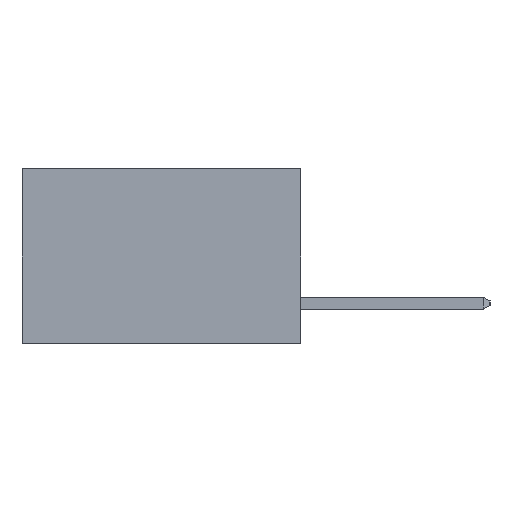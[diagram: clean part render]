
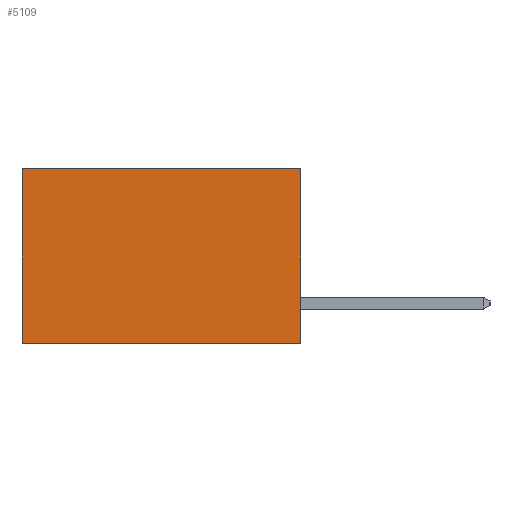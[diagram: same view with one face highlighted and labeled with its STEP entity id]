
A CAD part, left-side view. The second image highlights one B-rep face of the part: STEP entity #5109.
In plain terms, the highlighted planar face has unit normal (-1, 0, 0).
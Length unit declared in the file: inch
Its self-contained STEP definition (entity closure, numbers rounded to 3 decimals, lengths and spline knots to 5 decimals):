
#468 = DIRECTION ( 'NONE',  ( 0., 0., -1. ) ) ;
#529 = VERTEX_POINT ( 'NONE', #957 ) ;
#538 = DIRECTION ( 'NONE',  ( 1., 0., 0. ) ) ;
#957 = CARTESIAN_POINT ( 'NONE',  ( 0.277, 0.59, -0.37 ) ) ;
#1653 = LINE ( 'NONE', #14024, #4261 ) ;
#1787 = VERTEX_POINT ( 'NONE', #2367 ) ;
#1857 = LINE ( 'NONE', #8252, #10293 ) ;
#2367 = CARTESIAN_POINT ( 'NONE',  ( 0.277, 0., 0. ) ) ;
#2565 = CARTESIAN_POINT ( 'NONE',  ( 0.277, 0., -0.37 ) ) ;
#2618 = CARTESIAN_POINT ( 'NONE',  ( 0.277, 0., -0.37 ) ) ;
#3576 = EDGE_CURVE ( 'NONE', #7550, #529, #1653, .T. ) ;
#4092 = EDGE_CURVE ( 'NONE', #1787, #11605, #1857, .T. ) ;
#4261 = VECTOR ( 'NONE', #13981, 39.37008 ) ;
#4294 = DIRECTION ( 'NONE',  ( 0., 1., 0. ) ) ;
#4338 = EDGE_LOOP ( 'NONE', ( #12270, #10084, #7837, #12442 ) ) ;
#4370 = CARTESIAN_POINT ( 'NONE',  ( 0.277, 0., 0. ) ) ;
#4539 = EDGE_CURVE ( 'NONE', #1787, #7550, #10926, .T. ) ;
#4802 = VECTOR ( 'NONE', #4294, 39.37008 ) ;
#5109 = ADVANCED_FACE ( 'NONE', ( #13920 ), #5886, .F. ) ;
#5264 = AXIS2_PLACEMENT_3D ( 'NONE', #2618, #538, #468 ) ;
#5886 = PLANE ( 'NONE',  #5264 ) ;
#7550 = VERTEX_POINT ( 'NONE', #8222 ) ;
#7837 = ORIENTED_EDGE ( 'NONE', *, *, #4092, .F. ) ;
#8003 = DIRECTION ( 'NONE',  ( 0., 0., -1. ) ) ;
#8222 = CARTESIAN_POINT ( 'NONE',  ( 0.277, 0.59, 0. ) ) ;
#8252 = CARTESIAN_POINT ( 'NONE',  ( 0.277, 0., -0.37 ) ) ;
#9306 = DIRECTION ( 'NONE',  ( 0., 1., 0. ) ) ;
#10084 = ORIENTED_EDGE ( 'NONE', *, *, #11665, .F. ) ;
#10293 = VECTOR ( 'NONE', #8003, 39.37008 ) ;
#10926 = LINE ( 'NONE', #4370, #4802 ) ;
#11265 = LINE ( 'NONE', #12463, #13453 ) ;
#11605 = VERTEX_POINT ( 'NONE', #2565 ) ;
#11665 = EDGE_CURVE ( 'NONE', #11605, #529, #11265, .T. ) ;
#12270 = ORIENTED_EDGE ( 'NONE', *, *, #3576, .T. ) ;
#12442 = ORIENTED_EDGE ( 'NONE', *, *, #4539, .T. ) ;
#12463 = CARTESIAN_POINT ( 'NONE',  ( 0.277, 0., -0.37 ) ) ;
#13453 = VECTOR ( 'NONE', #9306, 39.37008 ) ;
#13920 = FACE_OUTER_BOUND ( 'NONE', #4338, .T. ) ;
#13981 = DIRECTION ( 'NONE',  ( 0., 0., -1. ) ) ;
#14024 = CARTESIAN_POINT ( 'NONE',  ( 0.277, 0.59, -0.37 ) ) ;
